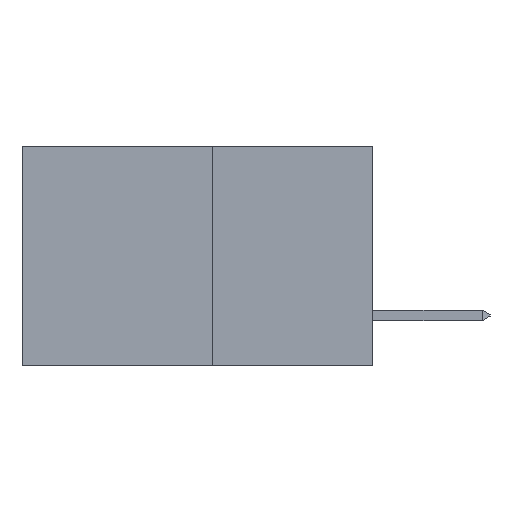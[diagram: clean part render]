
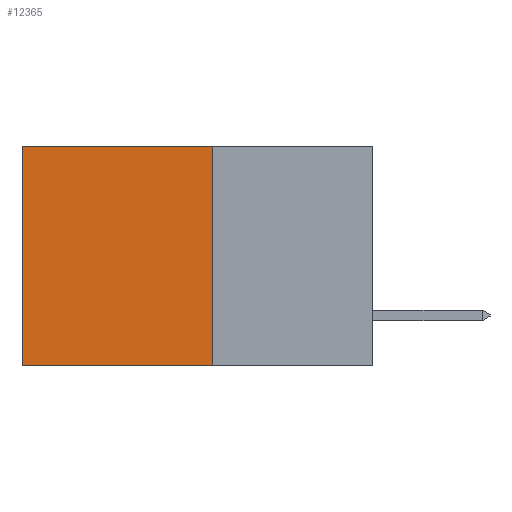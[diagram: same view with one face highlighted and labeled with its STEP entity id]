
A CAD part, left-side view. The second image highlights one B-rep face of the part: STEP entity #12365.
In plain terms, the highlighted planar face has unit normal (-1, 0, 0).
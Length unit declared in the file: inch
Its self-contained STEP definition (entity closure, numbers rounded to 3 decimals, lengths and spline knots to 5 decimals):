
#84 = ORIENTED_EDGE ( 'NONE', *, *, #23265, .F. ) ;
#1359 = DIRECTION ( 'NONE',  ( 0., 0., -1. ) ) ;
#2053 = DIRECTION ( 'NONE',  ( 1., 0., 0. ) ) ;
#2371 = ORIENTED_EDGE ( 'NONE', *, *, #18954, .T. ) ;
#3213 = EDGE_CURVE ( 'NONE', #8486, #10736, #29603, .T. ) ;
#3448 = VECTOR ( 'NONE', #1359, 39.37008 ) ;
#8486 = VERTEX_POINT ( 'NONE', #28086 ) ;
#8629 = DIRECTION ( 'NONE',  ( 0., 1., 0. ) ) ;
#9106 = LINE ( 'NONE', #15655, #3448 ) ;
#10736 = VERTEX_POINT ( 'NONE', #13315 ) ;
#12075 = DIRECTION ( 'NONE',  ( 0., 0., -1. ) ) ;
#12084 = ORIENTED_EDGE ( 'NONE', *, *, #23360, .T. ) ;
#12365 = ADVANCED_FACE ( 'NONE', ( #18161 ), #30307, .F. ) ;
#13315 = CARTESIAN_POINT ( 'NONE',  ( 0.277, 0.27, -0.37 ) ) ;
#15166 = VERTEX_POINT ( 'NONE', #28950 ) ;
#15182 = LINE ( 'NONE', #20352, #26905 ) ;
#15655 = CARTESIAN_POINT ( 'NONE',  ( 0.277, 0.59, -0.37 ) ) ;
#18161 = FACE_OUTER_BOUND ( 'NONE', #19745, .T. ) ;
#18276 = LINE ( 'NONE', #27017, #29974 ) ;
#18669 = DIRECTION ( 'NONE',  ( 0., 0., -1. ) ) ;
#18718 = VERTEX_POINT ( 'NONE', #21821 ) ;
#18954 = EDGE_CURVE ( 'NONE', #8486, #15166, #15182, .T. ) ;
#19745 = EDGE_LOOP ( 'NONE', ( #12084, #84, #20569, #2371 ) ) ;
#20352 = CARTESIAN_POINT ( 'NONE',  ( 0.277, 0.27, 0. ) ) ;
#20569 = ORIENTED_EDGE ( 'NONE', *, *, #3213, .F. ) ;
#20958 = CARTESIAN_POINT ( 'NONE',  ( 0.277, 0.27, -0.37 ) ) ;
#21821 = CARTESIAN_POINT ( 'NONE',  ( 0.277, 0.59, -0.37 ) ) ;
#23265 = EDGE_CURVE ( 'NONE', #10736, #18718, #18276, .T. ) ;
#23360 = EDGE_CURVE ( 'NONE', #15166, #18718, #9106, .T. ) ;
#24753 = DIRECTION ( 'NONE',  ( 0., 1., 0. ) ) ;
#25578 = CARTESIAN_POINT ( 'NONE',  ( 0.277, 0.27, -0.37 ) ) ;
#26905 = VECTOR ( 'NONE', #8629, 39.37008 ) ;
#27017 = CARTESIAN_POINT ( 'NONE',  ( 0.277, 0.27, -0.37 ) ) ;
#27107 = AXIS2_PLACEMENT_3D ( 'NONE', #20958, #2053, #18669 ) ;
#28086 = CARTESIAN_POINT ( 'NONE',  ( 0.277, 0.27, 0. ) ) ;
#28950 = CARTESIAN_POINT ( 'NONE',  ( 0.277, 0.59, 0. ) ) ;
#29603 = LINE ( 'NONE', #25578, #30331 ) ;
#29974 = VECTOR ( 'NONE', #24753, 39.37008 ) ;
#30307 = PLANE ( 'NONE',  #27107 ) ;
#30331 = VECTOR ( 'NONE', #12075, 39.37008 ) ;
